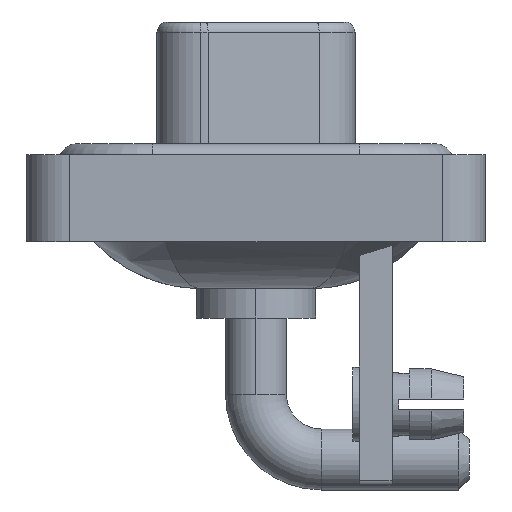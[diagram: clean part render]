
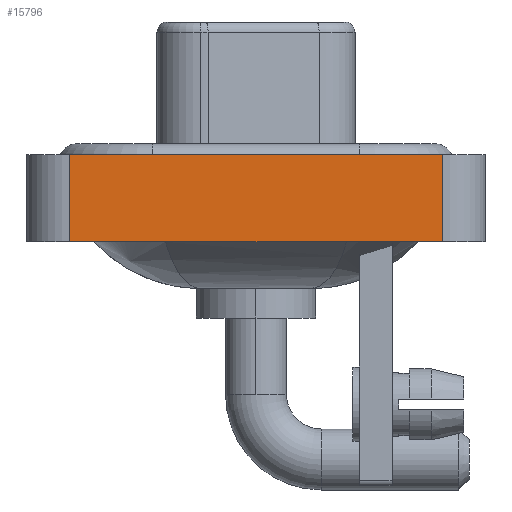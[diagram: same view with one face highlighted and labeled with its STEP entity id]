
A CAD part, left-side view. The second image highlights one B-rep face of the part: STEP entity #15796.
In plain terms, the highlighted planar face has unit normal (-1, 0, 0).
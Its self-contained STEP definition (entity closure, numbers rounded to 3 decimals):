
#111 = EDGE_CURVE ( 'NONE', #12133, #15320, #6511, .T. ) ;
#245 = VECTOR ( 'NONE', #7843, 1000. ) ;
#381 = FACE_OUTER_BOUND ( 'NONE', #16853, .T. ) ;
#1464 = DIRECTION ( 'NONE',  ( 0., -1., 0. ) ) ;
#1623 = AXIS2_PLACEMENT_3D ( 'NONE', #18103, #3703, #10668 ) ;
#1856 = DIRECTION ( 'NONE',  ( 0., 0., 1. ) ) ;
#3351 = CARTESIAN_POINT ( 'NONE',  ( -7.3, -8.55, 0.4 ) ) ;
#3703 = DIRECTION ( 'NONE',  ( -1., 0., 0. ) ) ;
#4012 = VERTEX_POINT ( 'NONE', #3351 ) ;
#5001 = CARTESIAN_POINT ( 'NONE',  ( -7.3, 8.55, -3.6 ) ) ;
#6511 = LINE ( 'NONE', #15105, #245 ) ;
#7024 = CARTESIAN_POINT ( 'NONE',  ( -7.3, 8.55, -3.6 ) ) ;
#7574 = ORIENTED_EDGE ( 'NONE', *, *, #111, .T. ) ;
#7843 = DIRECTION ( 'NONE',  ( 0., -1., 0. ) ) ;
#8386 = EDGE_CURVE ( 'NONE', #9224, #4012, #15522, .T. ) ;
#8441 = CARTESIAN_POINT ( 'NONE',  ( -7.3, -8.55, -3.6 ) ) ;
#8948 = ORIENTED_EDGE ( 'NONE', *, *, #9715, .F. ) ;
#9224 = VERTEX_POINT ( 'NONE', #13615 ) ;
#9715 = EDGE_CURVE ( 'NONE', #12133, #9224, #17897, .T. ) ;
#10133 = ORIENTED_EDGE ( 'NONE', *, *, #8386, .F. ) ;
#10668 = DIRECTION ( 'NONE',  ( 0., 0., 1. ) ) ;
#10916 = LINE ( 'NONE', #14929, #17436 ) ;
#12133 = VERTEX_POINT ( 'NONE', #7024 ) ;
#12382 = PLANE ( 'NONE',  #1623 ) ;
#12802 = VECTOR ( 'NONE', #1464, 1000. ) ;
#13615 = CARTESIAN_POINT ( 'NONE',  ( -7.3, 8.55, 0.4 ) ) ;
#14929 = CARTESIAN_POINT ( 'NONE',  ( -7.3, -8.55, -3.6 ) ) ;
#15105 = CARTESIAN_POINT ( 'NONE',  ( -7.3, -8.55, -3.6 ) ) ;
#15178 = EDGE_CURVE ( 'NONE', #15320, #4012, #10916, .T. ) ;
#15215 = DIRECTION ( 'NONE',  ( 0., 0., 1. ) ) ;
#15320 = VERTEX_POINT ( 'NONE', #8441 ) ;
#15522 = LINE ( 'NONE', #16943, #12802 ) ;
#15617 = VECTOR ( 'NONE', #15215, 1000. ) ;
#15796 = ADVANCED_FACE ( 'NONE', ( #381 ), #12382, .T. ) ;
#16853 = EDGE_LOOP ( 'NONE', ( #17474, #10133, #8948, #7574 ) ) ;
#16943 = CARTESIAN_POINT ( 'NONE',  ( -7.3, -8.55, 0.4 ) ) ;
#17436 = VECTOR ( 'NONE', #1856, 1000. ) ;
#17474 = ORIENTED_EDGE ( 'NONE', *, *, #15178, .T. ) ;
#17897 = LINE ( 'NONE', #5001, #15617 ) ;
#18103 = CARTESIAN_POINT ( 'NONE',  ( -7.3, -8.55, -3.6 ) ) ;
